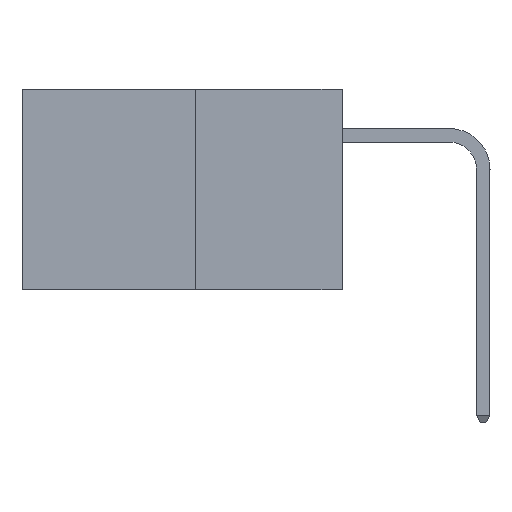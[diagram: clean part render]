
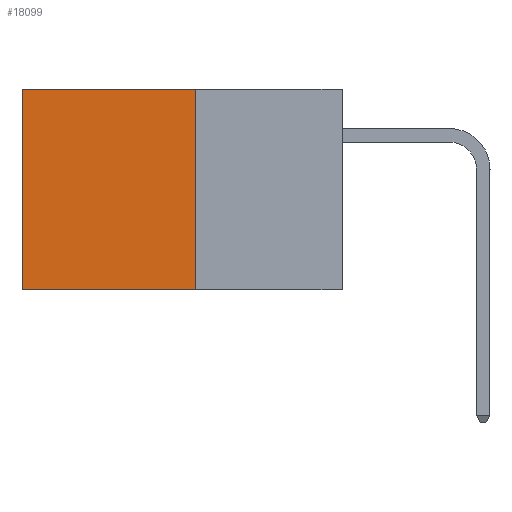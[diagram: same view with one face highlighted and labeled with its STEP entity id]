
A CAD part, left-side view. The second image highlights one B-rep face of the part: STEP entity #18099.
In plain terms, the highlighted planar face has unit normal (-1, 0, 0).
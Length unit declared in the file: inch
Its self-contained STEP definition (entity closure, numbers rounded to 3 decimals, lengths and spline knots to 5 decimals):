
#22 = CARTESIAN_POINT ( 'NONE',  ( 0.277, 0.27, -0.37 ) ) ;
#37 = CARTESIAN_POINT ( 'NONE',  ( 0.277, 0.27, 0. ) ) ;
#348 = CARTESIAN_POINT ( 'NONE',  ( 0.277, 0.59, 0. ) ) ;
#752 = DIRECTION ( 'NONE',  ( 1., 0., 0. ) ) ;
#1210 = EDGE_CURVE ( 'NONE', #4230, #7538, #9354, .T. ) ;
#1737 = DIRECTION ( 'NONE',  ( 0., 0., -1. ) ) ;
#1934 = VECTOR ( 'NONE', #11561, 39.37008 ) ;
#4217 = VECTOR ( 'NONE', #1737, 39.37008 ) ;
#4230 = VERTEX_POINT ( 'NONE', #5289 ) ;
#4857 = FACE_OUTER_BOUND ( 'NONE', #12006, .T. ) ;
#5289 = CARTESIAN_POINT ( 'NONE',  ( 0.277, 0.27, -0.37 ) ) ;
#5583 = ORIENTED_EDGE ( 'NONE', *, *, #20588, .F. ) ;
#5937 = VERTEX_POINT ( 'NONE', #37 ) ;
#5997 = CARTESIAN_POINT ( 'NONE',  ( 0.277, 0.59, -0.37 ) ) ;
#7377 = CARTESIAN_POINT ( 'NONE',  ( 0.277, 0.27, 0. ) ) ;
#7538 = VERTEX_POINT ( 'NONE', #5997 ) ;
#7922 = VECTOR ( 'NONE', #18943, 39.37008 ) ;
#8359 = ORIENTED_EDGE ( 'NONE', *, *, #18779, .T. ) ;
#8455 = LINE ( 'NONE', #7377, #7922 ) ;
#8991 = ORIENTED_EDGE ( 'NONE', *, *, #1210, .F. ) ;
#9091 = VERTEX_POINT ( 'NONE', #348 ) ;
#9354 = LINE ( 'NONE', #19598, #13783 ) ;
#10776 = CARTESIAN_POINT ( 'NONE',  ( 0.277, 0.27, -0.37 ) ) ;
#11326 = LINE ( 'NONE', #14899, #1934 ) ;
#11561 = DIRECTION ( 'NONE',  ( 0., 0., -1. ) ) ;
#12006 = EDGE_LOOP ( 'NONE', ( #17801, #8991, #5583, #8359 ) ) ;
#12458 = DIRECTION ( 'NONE',  ( 0., 0., -1. ) ) ;
#12575 = AXIS2_PLACEMENT_3D ( 'NONE', #10776, #752, #12458 ) ;
#13783 = VECTOR ( 'NONE', #17194, 39.37008 ) ;
#14899 = CARTESIAN_POINT ( 'NONE',  ( 0.277, 0.59, -0.37 ) ) ;
#17194 = DIRECTION ( 'NONE',  ( 0., 1., 0. ) ) ;
#17413 = LINE ( 'NONE', #22, #4217 ) ;
#17801 = ORIENTED_EDGE ( 'NONE', *, *, #18430, .T. ) ;
#18099 = ADVANCED_FACE ( 'NONE', ( #4857 ), #20587, .F. ) ;
#18430 = EDGE_CURVE ( 'NONE', #9091, #7538, #11326, .T. ) ;
#18779 = EDGE_CURVE ( 'NONE', #5937, #9091, #8455, .T. ) ;
#18943 = DIRECTION ( 'NONE',  ( 0., 1., 0. ) ) ;
#19598 = CARTESIAN_POINT ( 'NONE',  ( 0.277, 0.27, -0.37 ) ) ;
#20587 = PLANE ( 'NONE',  #12575 ) ;
#20588 = EDGE_CURVE ( 'NONE', #5937, #4230, #17413, .T. ) ;
